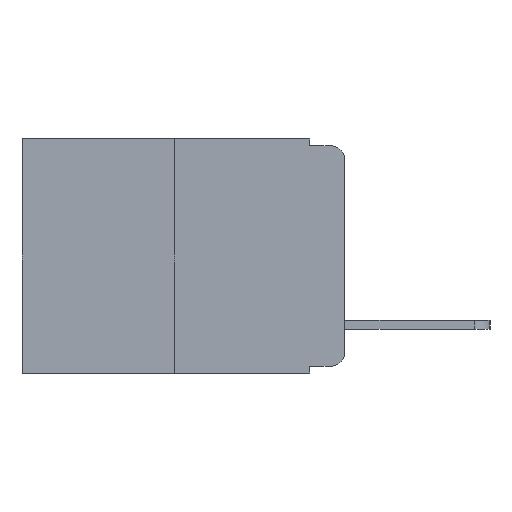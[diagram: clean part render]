
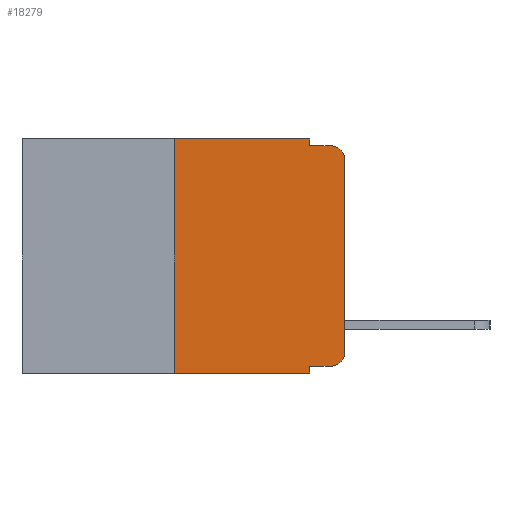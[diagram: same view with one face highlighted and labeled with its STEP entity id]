
A CAD part, left-side view. The second image highlights one B-rep face of the part: STEP entity #18279.
In plain terms, the highlighted planar face has unit normal (-1, 0, 0).
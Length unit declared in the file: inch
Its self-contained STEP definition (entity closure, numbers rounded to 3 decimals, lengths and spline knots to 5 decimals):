
#585 = LINE ( 'NONE', #17983, #6464 ) ;
#615 = VERTEX_POINT ( 'NONE', #8453 ) ;
#1045 = VECTOR ( 'NONE', #3125, 39.37008 ) ;
#1933 = ORIENTED_EDGE ( 'NONE', *, *, #17265, .F. ) ;
#1959 = VERTEX_POINT ( 'NONE', #5793 ) ;
#2399 = VERTEX_POINT ( 'NONE', #19778 ) ;
#2682 = EDGE_CURVE ( 'NONE', #615, #2399, #19771, .T. ) ;
#3125 = DIRECTION ( 'NONE',  ( 0., 0., -1. ) ) ;
#3238 = CARTESIAN_POINT ( 'NONE',  ( 0., 0.051, 0. ) ) ;
#3638 = ORIENTED_EDGE ( 'NONE', *, *, #2682, .T. ) ;
#3721 = EDGE_CURVE ( 'NONE', #15418, #13702, #9842, .T. ) ;
#3773 = CARTESIAN_POINT ( 'NONE',  ( 0., 0.25, 0. ) ) ;
#3900 = CIRCLE ( 'NONE', #17061, 0.02 ) ;
#4176 = ORIENTED_EDGE ( 'NONE', *, *, #6058, .T. ) ;
#4253 = DIRECTION ( 'NONE',  ( 0., 0., -1. ) ) ;
#4351 = EDGE_LOOP ( 'NONE', ( #21638, #8735, #14999, #10851, #9385, #18250, #15194, #1933, #4176, #3638 ) ) ;
#4887 = CARTESIAN_POINT ( 'NONE',  ( 0., 0., -0.03 ) ) ;
#5793 = CARTESIAN_POINT ( 'NONE',  ( 0., 0.051, -0.01 ) ) ;
#5850 = PLANE ( 'NONE',  #14974 ) ;
#5853 = DIRECTION ( 'NONE',  ( 0., 0., -1. ) ) ;
#6058 = EDGE_CURVE ( 'NONE', #15592, #615, #17502, .T. ) ;
#6116 = CARTESIAN_POINT ( 'NONE',  ( 0., 0.051, 0. ) ) ;
#6288 = VERTEX_POINT ( 'NONE', #4887 ) ;
#6464 = VECTOR ( 'NONE', #19446, 39.37008 ) ;
#7039 = VERTEX_POINT ( 'NONE', #19052 ) ;
#7513 = CARTESIAN_POINT ( 'NONE',  ( 0., 0.25, -0.343 ) ) ;
#7699 = CARTESIAN_POINT ( 'NONE',  ( 0., 0.051, 0. ) ) ;
#8145 = LINE ( 'NONE', #7699, #19245 ) ;
#8259 = LINE ( 'NONE', #15028, #19098 ) ;
#8310 = LINE ( 'NONE', #13070, #16408 ) ;
#8453 = CARTESIAN_POINT ( 'NONE',  ( 0., 0.02, -0.333 ) ) ;
#8735 = ORIENTED_EDGE ( 'NONE', *, *, #14299, .T. ) ;
#8746 = AXIS2_PLACEMENT_3D ( 'NONE', #12701, #17552, #5853 ) ;
#9258 = DIRECTION ( 'NONE',  ( 1., 0., 0. ) ) ;
#9385 = ORIENTED_EDGE ( 'NONE', *, *, #11985, .F. ) ;
#9842 = LINE ( 'NONE', #11735, #15017 ) ;
#9991 = LINE ( 'NONE', #10941, #20395 ) ;
#10851 = ORIENTED_EDGE ( 'NONE', *, *, #17084, .F. ) ;
#10941 = CARTESIAN_POINT ( 'NONE',  ( 0., 0.473, -0.343 ) ) ;
#11377 = CARTESIAN_POINT ( 'NONE',  ( 0., 0.051, -0.333 ) ) ;
#11735 = CARTESIAN_POINT ( 'NONE',  ( 0., 0.25, 0. ) ) ;
#11985 = EDGE_CURVE ( 'NONE', #13702, #18890, #8259, .T. ) ;
#12701 = CARTESIAN_POINT ( 'NONE',  ( 0., 0.02, -0.313 ) ) ;
#12746 = CARTESIAN_POINT ( 'NONE',  ( 0., 0.02, -0.01 ) ) ;
#12933 = DIRECTION ( 'NONE',  ( 0., -1., 0. ) ) ;
#13070 = CARTESIAN_POINT ( 'NONE',  ( 0., 0., 0. ) ) ;
#13460 = LINE ( 'NONE', #3238, #1045 ) ;
#13702 = VERTEX_POINT ( 'NONE', #3773 ) ;
#14299 = EDGE_CURVE ( 'NONE', #6288, #16278, #3900, .T. ) ;
#14719 = DIRECTION ( 'NONE',  ( -1., 0., 0. ) ) ;
#14901 = DIRECTION ( 'NONE',  ( 0., 0., -1. ) ) ;
#14974 = AXIS2_PLACEMENT_3D ( 'NONE', #19432, #9258, #4253 ) ;
#14999 = ORIENTED_EDGE ( 'NONE', *, *, #19678, .F. ) ;
#15017 = VECTOR ( 'NONE', #21560, 39.37008 ) ;
#15028 = CARTESIAN_POINT ( 'NONE',  ( 0., 0.473, 0. ) ) ;
#15194 = ORIENTED_EDGE ( 'NONE', *, *, #20884, .T. ) ;
#15418 = VERTEX_POINT ( 'NONE', #7513 ) ;
#15592 = VERTEX_POINT ( 'NONE', #11377 ) ;
#16142 = CARTESIAN_POINT ( 'NONE',  ( 0., 0.051, -0.333 ) ) ;
#16278 = VERTEX_POINT ( 'NONE', #12746 ) ;
#16408 = VECTOR ( 'NONE', #21460, 39.37008 ) ;
#16418 = EDGE_CURVE ( 'NONE', #2399, #6288, #8310, .T. ) ;
#17061 = AXIS2_PLACEMENT_3D ( 'NONE', #21437, #14719, #21552 ) ;
#17084 = EDGE_CURVE ( 'NONE', #18890, #1959, #8145, .T. ) ;
#17265 = EDGE_CURVE ( 'NONE', #15592, #7039, #13460, .T. ) ;
#17502 = LINE ( 'NONE', #16142, #17646 ) ;
#17552 = DIRECTION ( 'NONE',  ( -1., 0., 0. ) ) ;
#17646 = VECTOR ( 'NONE', #19169, 39.37008 ) ;
#17983 = CARTESIAN_POINT ( 'NONE',  ( 0., 0.051, -0.01 ) ) ;
#18250 = ORIENTED_EDGE ( 'NONE', *, *, #3721, .F. ) ;
#18279 = ADVANCED_FACE ( 'NONE', ( #20768 ), #5850, .F. ) ;
#18890 = VERTEX_POINT ( 'NONE', #6116 ) ;
#19052 = CARTESIAN_POINT ( 'NONE',  ( 0., 0.051, -0.343 ) ) ;
#19098 = VECTOR ( 'NONE', #21851, 39.37008 ) ;
#19169 = DIRECTION ( 'NONE',  ( 0., -1., 0. ) ) ;
#19245 = VECTOR ( 'NONE', #14901, 39.37008 ) ;
#19432 = CARTESIAN_POINT ( 'NONE',  ( 0., 0.473, 0. ) ) ;
#19446 = DIRECTION ( 'NONE',  ( 0., -1., 0. ) ) ;
#19678 = EDGE_CURVE ( 'NONE', #1959, #16278, #585, .T. ) ;
#19771 = CIRCLE ( 'NONE', #8746, 0.02 ) ;
#19778 = CARTESIAN_POINT ( 'NONE',  ( 0., 0., -0.313 ) ) ;
#20395 = VECTOR ( 'NONE', #12933, 39.37008 ) ;
#20768 = FACE_OUTER_BOUND ( 'NONE', #4351, .T. ) ;
#20884 = EDGE_CURVE ( 'NONE', #15418, #7039, #9991, .T. ) ;
#21437 = CARTESIAN_POINT ( 'NONE',  ( 0., 0.02, -0.03 ) ) ;
#21460 = DIRECTION ( 'NONE',  ( 0., 0., 1. ) ) ;
#21552 = DIRECTION ( 'NONE',  ( 0., 0., -1. ) ) ;
#21560 = DIRECTION ( 'NONE',  ( 0., 0., 1. ) ) ;
#21638 = ORIENTED_EDGE ( 'NONE', *, *, #16418, .T. ) ;
#21851 = DIRECTION ( 'NONE',  ( 0., -1., 0. ) ) ;
